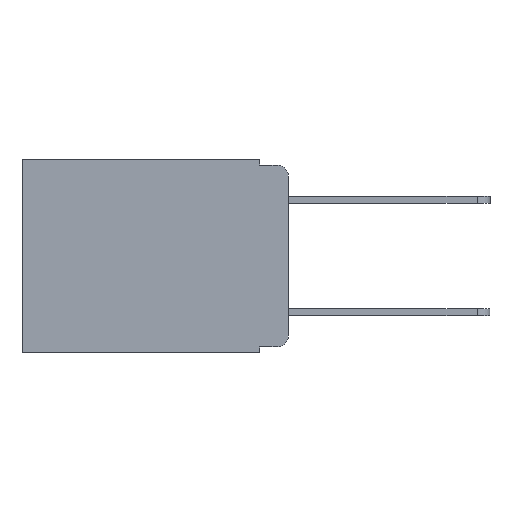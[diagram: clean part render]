
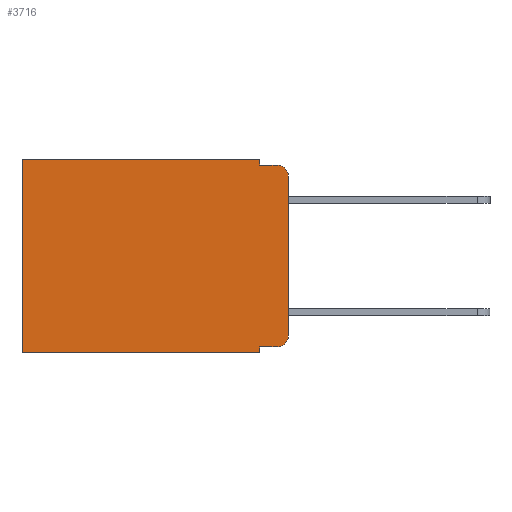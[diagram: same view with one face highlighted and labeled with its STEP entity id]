
A CAD part, left-side view. The second image highlights one B-rep face of the part: STEP entity #3716.
In plain terms, the highlighted planar face has unit normal (-1, 0, 0).
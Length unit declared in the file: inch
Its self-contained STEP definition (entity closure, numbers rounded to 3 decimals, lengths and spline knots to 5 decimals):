
#32 = CARTESIAN_POINT ( 'NONE',  ( 0.298, 0., 0. ) ) ;
#102 = ORIENTED_EDGE ( 'NONE', *, *, #811, .T. ) ;
#231 = EDGE_CURVE ( 'NONE', #5985, #5996, #6173, .T. ) ;
#320 = VERTEX_POINT ( 'NONE', #2963 ) ;
#412 = CARTESIAN_POINT ( 'NONE',  ( 0.298, 0.051, -0.343 ) ) ;
#456 = CARTESIAN_POINT ( 'NONE',  ( 0.298, 0.02, -0.01 ) ) ;
#740 = VECTOR ( 'NONE', #2255, 39.37008 ) ;
#811 = EDGE_CURVE ( 'NONE', #5996, #3620, #5235, .T. ) ;
#949 = VECTOR ( 'NONE', #8656, 39.37008 ) ;
#1046 = DIRECTION ( 'NONE',  ( 0., 0., -1. ) ) ;
#1197 = DIRECTION ( 'NONE',  ( 0., 0., -1. ) ) ;
#1285 = DIRECTION ( 'NONE',  ( -1., 0., 0. ) ) ;
#1287 = CARTESIAN_POINT ( 'NONE',  ( 0.298, 0.02, -0.03 ) ) ;
#1364 = EDGE_CURVE ( 'NONE', #5985, #9309, #4126, .T. ) ;
#1385 = VECTOR ( 'NONE', #7484, 39.37008 ) ;
#1394 = VERTEX_POINT ( 'NONE', #4529 ) ;
#1457 = VERTEX_POINT ( 'NONE', #8531 ) ;
#1593 = DIRECTION ( 'NONE',  ( 0., 0., -1. ) ) ;
#1900 = EDGE_CURVE ( 'NONE', #9745, #1394, #2115, .T. ) ;
#1943 = VERTEX_POINT ( 'NONE', #2904 ) ;
#2115 = LINE ( 'NONE', #2153, #9824 ) ;
#2153 = CARTESIAN_POINT ( 'NONE',  ( 0.298, 0.473, 0. ) ) ;
#2255 = DIRECTION ( 'NONE',  ( 0., 1., 0. ) ) ;
#2561 = VECTOR ( 'NONE', #3332, 39.37008 ) ;
#2796 = LINE ( 'NONE', #9270, #949 ) ;
#2837 = AXIS2_PLACEMENT_3D ( 'NONE', #5584, #3966, #4982 ) ;
#2904 = CARTESIAN_POINT ( 'NONE',  ( 0.298, 0.051, -0.01 ) ) ;
#2930 = EDGE_CURVE ( 'NONE', #1457, #1943, #4995, .T. ) ;
#2963 = CARTESIAN_POINT ( 'NONE',  ( 0.298, 0., -0.03 ) ) ;
#3114 = CARTESIAN_POINT ( 'NONE',  ( 0.298, 0., -0.343 ) ) ;
#3332 = DIRECTION ( 'NONE',  ( 0., 0., -1. ) ) ;
#3381 = EDGE_CURVE ( 'NONE', #320, #3620, #9252, .T. ) ;
#3492 = EDGE_CURVE ( 'NONE', #1943, #7271, #2796, .T. ) ;
#3620 = VERTEX_POINT ( 'NONE', #6548 ) ;
#3716 = ADVANCED_FACE ( 'NONE', ( #9143 ), #7988, .F. ) ;
#3784 = CARTESIAN_POINT ( 'NONE',  ( 0.298, 0.051, 0. ) ) ;
#3802 = CARTESIAN_POINT ( 'NONE',  ( 0.298, 0.473, 0. ) ) ;
#3966 = DIRECTION ( 'NONE',  ( -1., 0., 0. ) ) ;
#3980 = ORIENTED_EDGE ( 'NONE', *, *, #3381, .F. ) ;
#3995 = ORIENTED_EDGE ( 'NONE', *, *, #1364, .F. ) ;
#4126 = LINE ( 'NONE', #8740, #7553 ) ;
#4291 = ORIENTED_EDGE ( 'NONE', *, *, #3492, .F. ) ;
#4529 = CARTESIAN_POINT ( 'NONE',  ( 0.298, 0.473, -0.343 ) ) ;
#4654 = VECTOR ( 'NONE', #8904, 39.37008 ) ;
#4829 = ORIENTED_EDGE ( 'NONE', *, *, #231, .T. ) ;
#4842 = AXIS2_PLACEMENT_3D ( 'NONE', #1287, #1285, #1593 ) ;
#4982 = DIRECTION ( 'NONE',  ( 0., 0., -1. ) ) ;
#4995 = LINE ( 'NONE', #3784, #2561 ) ;
#5235 = CIRCLE ( 'NONE', #2837, 0.02 ) ;
#5584 = CARTESIAN_POINT ( 'NONE',  ( 0.298, 0.02, -0.313 ) ) ;
#5985 = VERTEX_POINT ( 'NONE', #7470 ) ;
#5996 = VERTEX_POINT ( 'NONE', #9500 ) ;
#6097 = CARTESIAN_POINT ( 'NONE',  ( 0.298, 0.051, -0.333 ) ) ;
#6173 = LINE ( 'NONE', #6097, #4654 ) ;
#6261 = EDGE_CURVE ( 'NONE', #9309, #1394, #7264, .T. ) ;
#6462 = ORIENTED_EDGE ( 'NONE', *, *, #1900, .T. ) ;
#6548 = CARTESIAN_POINT ( 'NONE',  ( 0.298, 0., -0.313 ) ) ;
#6608 = DIRECTION ( 'NONE',  ( 1., 0., 0. ) ) ;
#6620 = CIRCLE ( 'NONE', #4842, 0.02 ) ;
#6672 = CARTESIAN_POINT ( 'NONE',  ( 0.298, 0., 0. ) ) ;
#6925 = AXIS2_PLACEMENT_3D ( 'NONE', #6672, #6608, #9314 ) ;
#6926 = ORIENTED_EDGE ( 'NONE', *, *, #6261, .F. ) ;
#7096 = ORIENTED_EDGE ( 'NONE', *, *, #7811, .T. ) ;
#7165 = LINE ( 'NONE', #7410, #740 ) ;
#7168 = ORIENTED_EDGE ( 'NONE', *, *, #8540, .T. ) ;
#7264 = LINE ( 'NONE', #3114, #1385 ) ;
#7271 = VERTEX_POINT ( 'NONE', #456 ) ;
#7365 = ORIENTED_EDGE ( 'NONE', *, *, #2930, .F. ) ;
#7410 = CARTESIAN_POINT ( 'NONE',  ( 0.298, 0., 0. ) ) ;
#7470 = CARTESIAN_POINT ( 'NONE',  ( 0.298, 0.051, -0.333 ) ) ;
#7484 = DIRECTION ( 'NONE',  ( 0., 1., 0. ) ) ;
#7537 = VECTOR ( 'NONE', #1046, 39.37008 ) ;
#7553 = VECTOR ( 'NONE', #1197, 39.37008 ) ;
#7568 = DIRECTION ( 'NONE',  ( 0., 0., -1. ) ) ;
#7811 = EDGE_CURVE ( 'NONE', #320, #7271, #6620, .T. ) ;
#7988 = PLANE ( 'NONE',  #6925 ) ;
#8531 = CARTESIAN_POINT ( 'NONE',  ( 0.298, 0.051, 0. ) ) ;
#8540 = EDGE_CURVE ( 'NONE', #1457, #9745, #7165, .T. ) ;
#8656 = DIRECTION ( 'NONE',  ( 0., -1., 0. ) ) ;
#8740 = CARTESIAN_POINT ( 'NONE',  ( 0.298, 0.051, 0. ) ) ;
#8846 = EDGE_LOOP ( 'NONE', ( #3980, #7096, #4291, #7365, #7168, #6462, #6926, #3995, #4829, #102 ) ) ;
#8904 = DIRECTION ( 'NONE',  ( 0., -1., 0. ) ) ;
#9143 = FACE_OUTER_BOUND ( 'NONE', #8846, .T. ) ;
#9252 = LINE ( 'NONE', #32, #7537 ) ;
#9270 = CARTESIAN_POINT ( 'NONE',  ( 0.298, 0.051, -0.01 ) ) ;
#9309 = VERTEX_POINT ( 'NONE', #412 ) ;
#9314 = DIRECTION ( 'NONE',  ( 0., 0., -1. ) ) ;
#9500 = CARTESIAN_POINT ( 'NONE',  ( 0.298, 0.02, -0.333 ) ) ;
#9745 = VERTEX_POINT ( 'NONE', #3802 ) ;
#9824 = VECTOR ( 'NONE', #7568, 39.37008 ) ;
